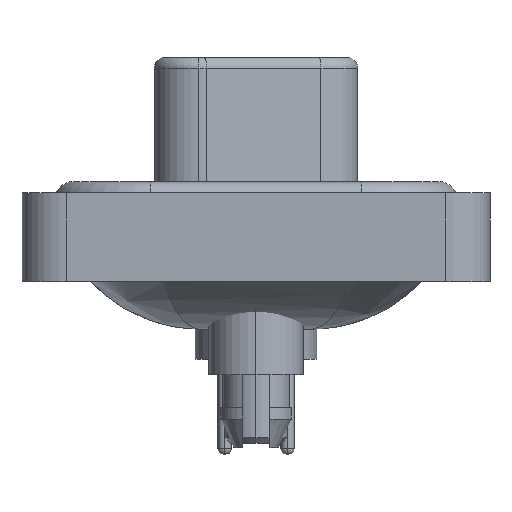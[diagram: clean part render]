
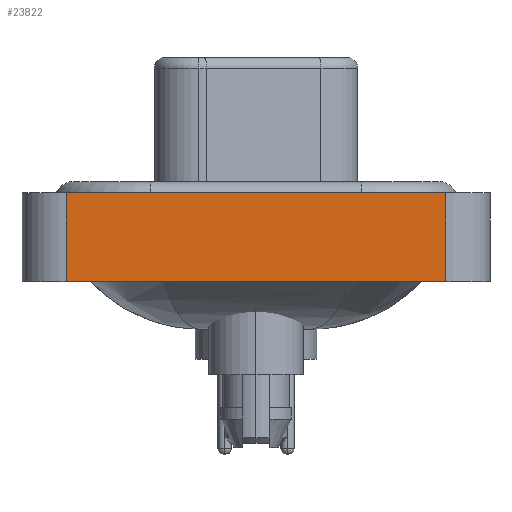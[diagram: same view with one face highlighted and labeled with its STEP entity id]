
A CAD part, left-side view. The second image highlights one B-rep face of the part: STEP entity #23822.
In plain terms, the highlighted planar face has unit normal (-1, 0, 0).
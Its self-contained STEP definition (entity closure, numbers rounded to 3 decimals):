
#1131 = CARTESIAN_POINT ( 'NONE',  ( -7.3, 8.55, -3.6 ) ) ;
#2460 = ORIENTED_EDGE ( 'NONE', *, *, #18097, .F. ) ;
#2570 = EDGE_CURVE ( 'NONE', #4936, #7868, #24080, .T. ) ;
#3277 = VECTOR ( 'NONE', #20942, 1000. ) ;
#3419 = DIRECTION ( 'NONE',  ( 0., -1., 0. ) ) ;
#3759 = CARTESIAN_POINT ( 'NONE',  ( -7.3, -8.55, -3.6 ) ) ;
#3833 = CARTESIAN_POINT ( 'NONE',  ( -7.3, 8.55, 0.4 ) ) ;
#4936 = VERTEX_POINT ( 'NONE', #1131 ) ;
#6504 = ORIENTED_EDGE ( 'NONE', *, *, #2570, .T. ) ;
#6528 = VERTEX_POINT ( 'NONE', #3833 ) ;
#7306 = DIRECTION ( 'NONE',  ( 0., 0., 1. ) ) ;
#7428 = LINE ( 'NONE', #14948, #20231 ) ;
#7854 = ORIENTED_EDGE ( 'NONE', *, *, #21312, .F. ) ;
#7868 = VERTEX_POINT ( 'NONE', #10860 ) ;
#9726 = DIRECTION ( 'NONE',  ( -1., 0., 0. ) ) ;
#10860 = CARTESIAN_POINT ( 'NONE',  ( -7.3, -8.55, -3.6 ) ) ;
#11587 = PLANE ( 'NONE',  #13446 ) ;
#11866 = DIRECTION ( 'NONE',  ( 0., -1., 0. ) ) ;
#12507 = EDGE_CURVE ( 'NONE', #7868, #14304, #20702, .T. ) ;
#13446 = AXIS2_PLACEMENT_3D ( 'NONE', #21370, #9726, #21484 ) ;
#13610 = EDGE_LOOP ( 'NONE', ( #19970, #2460, #7854, #6504 ) ) ;
#14304 = VERTEX_POINT ( 'NONE', #22611 ) ;
#14751 = CARTESIAN_POINT ( 'NONE',  ( -7.3, -8.55, -3.6 ) ) ;
#14948 = CARTESIAN_POINT ( 'NONE',  ( -7.3, 8.55, -3.6 ) ) ;
#17511 = LINE ( 'NONE', #19222, #18335 ) ;
#18039 = VECTOR ( 'NONE', #3419, 1000. ) ;
#18097 = EDGE_CURVE ( 'NONE', #6528, #14304, #17511, .T. ) ;
#18335 = VECTOR ( 'NONE', #11866, 1000. ) ;
#19222 = CARTESIAN_POINT ( 'NONE',  ( -7.3, -8.55, 0.4 ) ) ;
#19970 = ORIENTED_EDGE ( 'NONE', *, *, #12507, .T. ) ;
#20231 = VECTOR ( 'NONE', #7306, 1000. ) ;
#20702 = LINE ( 'NONE', #3759, #3277 ) ;
#20942 = DIRECTION ( 'NONE',  ( 0., 0., 1. ) ) ;
#21312 = EDGE_CURVE ( 'NONE', #4936, #6528, #7428, .T. ) ;
#21370 = CARTESIAN_POINT ( 'NONE',  ( -7.3, -8.55, -3.6 ) ) ;
#21484 = DIRECTION ( 'NONE',  ( 0., 0., 1. ) ) ;
#22611 = CARTESIAN_POINT ( 'NONE',  ( -7.3, -8.55, 0.4 ) ) ;
#23583 = FACE_OUTER_BOUND ( 'NONE', #13610, .T. ) ;
#23822 = ADVANCED_FACE ( 'NONE', ( #23583 ), #11587, .T. ) ;
#24080 = LINE ( 'NONE', #14751, #18039 ) ;
